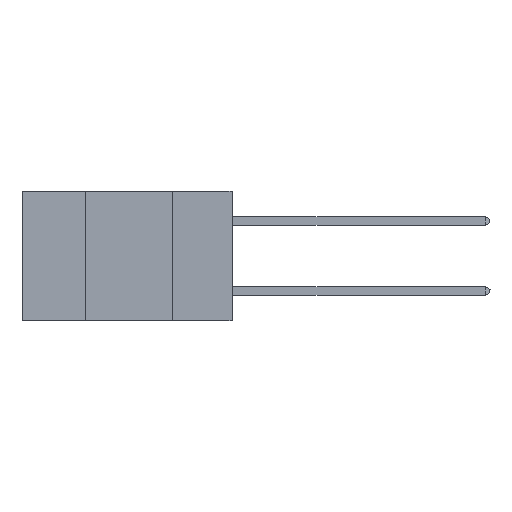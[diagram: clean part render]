
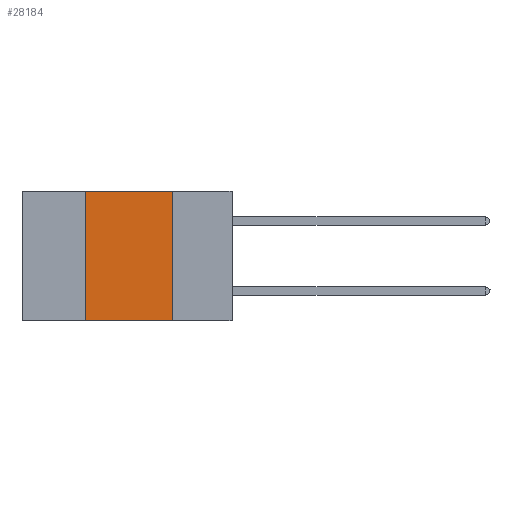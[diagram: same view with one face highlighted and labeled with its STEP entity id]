
A CAD part, left-side view. The second image highlights one B-rep face of the part: STEP entity #28184.
In plain terms, the highlighted planar face has unit normal (-1, 0, 0).
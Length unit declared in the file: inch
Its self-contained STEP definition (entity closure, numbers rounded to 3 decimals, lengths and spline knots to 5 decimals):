
#127 = EDGE_LOOP ( 'NONE', ( #11099, #27451, #23113, #28710 ) ) ;
#2612 = PLANE ( 'NONE',  #22854 ) ;
#4253 = CARTESIAN_POINT ( 'NONE',  ( 0., 0.17, 0. ) ) ;
#4783 = CARTESIAN_POINT ( 'NONE',  ( 0., 0.6, 0. ) ) ;
#5740 = CARTESIAN_POINT ( 'NONE',  ( 0., 0.6, -0.37 ) ) ;
#6977 = DIRECTION ( 'NONE',  ( 0., 0., 1. ) ) ;
#7565 = CARTESIAN_POINT ( 'NONE',  ( 0., 0.17, -0.37 ) ) ;
#8436 = VERTEX_POINT ( 'NONE', #4253 ) ;
#9278 = EDGE_CURVE ( 'NONE', #8436, #23291, #13186, .T. ) ;
#9604 = DIRECTION ( 'NONE',  ( 0., -1., 0. ) ) ;
#10178 = DIRECTION ( 'NONE',  ( 0., 0., -1. ) ) ;
#10862 = EDGE_CURVE ( 'NONE', #26704, #23291, #21529, .T. ) ;
#10948 = EDGE_CURVE ( 'NONE', #26704, #12681, #19699, .T. ) ;
#11004 = VECTOR ( 'NONE', #9604, 39.37008 ) ;
#11099 = ORIENTED_EDGE ( 'NONE', *, *, #9278, .F. ) ;
#12145 = EDGE_CURVE ( 'NONE', #12681, #8436, #21821, .T. ) ;
#12681 = VERTEX_POINT ( 'NONE', #15904 ) ;
#13186 = LINE ( 'NONE', #23984, #14259 ) ;
#14259 = VECTOR ( 'NONE', #10178, 39.37008 ) ;
#14330 = DIRECTION ( 'NONE',  ( 0., 0., -1. ) ) ;
#15362 = VECTOR ( 'NONE', #6977, 39.37008 ) ;
#15390 = VECTOR ( 'NONE', #22660, 39.37008 ) ;
#15904 = CARTESIAN_POINT ( 'NONE',  ( 0., 0.42, 0. ) ) ;
#16045 = FACE_OUTER_BOUND ( 'NONE', #127, .T. ) ;
#19699 = LINE ( 'NONE', #29502, #15362 ) ;
#21529 = LINE ( 'NONE', #5740, #15390 ) ;
#21821 = LINE ( 'NONE', #4783, #11004 ) ;
#22660 = DIRECTION ( 'NONE',  ( 0., -1., 0. ) ) ;
#22854 = AXIS2_PLACEMENT_3D ( 'NONE', #25912, #26006, #14330 ) ;
#23113 = ORIENTED_EDGE ( 'NONE', *, *, #10948, .F. ) ;
#23291 = VERTEX_POINT ( 'NONE', #7565 ) ;
#23984 = CARTESIAN_POINT ( 'NONE',  ( 0., 0.17, 0. ) ) ;
#25912 = CARTESIAN_POINT ( 'NONE',  ( 0., 0.6, 0. ) ) ;
#26006 = DIRECTION ( 'NONE',  ( 1., 0., 0. ) ) ;
#26704 = VERTEX_POINT ( 'NONE', #29763 ) ;
#27451 = ORIENTED_EDGE ( 'NONE', *, *, #12145, .F. ) ;
#28184 = ADVANCED_FACE ( 'NONE', ( #16045 ), #2612, .F. ) ;
#28710 = ORIENTED_EDGE ( 'NONE', *, *, #10862, .T. ) ;
#29502 = CARTESIAN_POINT ( 'NONE',  ( 0., 0.42, 0. ) ) ;
#29763 = CARTESIAN_POINT ( 'NONE',  ( 0., 0.42, -0.37 ) ) ;
